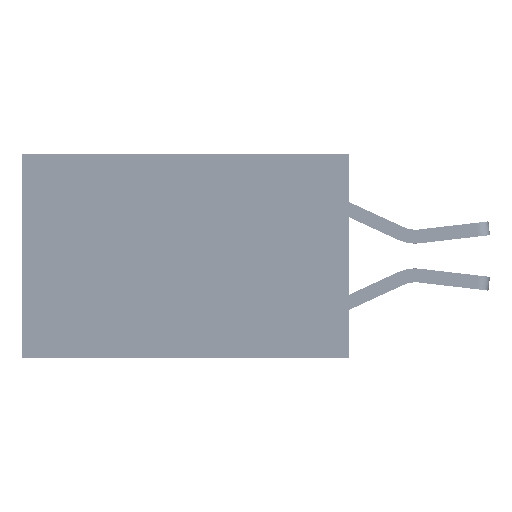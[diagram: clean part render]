
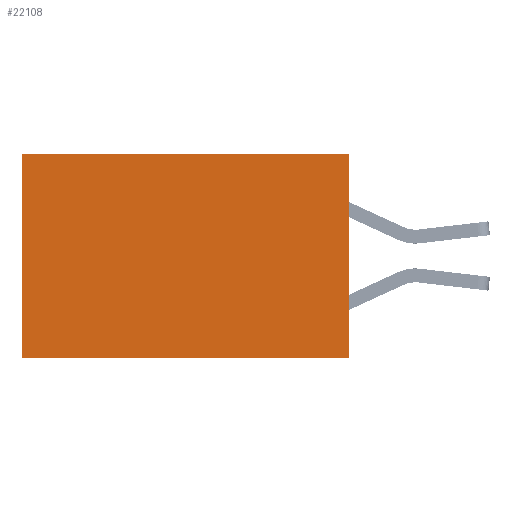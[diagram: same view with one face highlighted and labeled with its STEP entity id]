
A CAD part, left-side view. The second image highlights one B-rep face of the part: STEP entity #22108.
In plain terms, the highlighted planar face has unit normal (-1, 0, 0).
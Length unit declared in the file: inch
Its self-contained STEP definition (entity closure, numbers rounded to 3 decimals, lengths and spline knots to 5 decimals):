
#713 = CARTESIAN_POINT ( 'NONE',  ( 0.277, 0., -0.37 ) ) ;
#821 = DIRECTION ( 'NONE',  ( 0., 0., -1. ) ) ;
#1561 = CARTESIAN_POINT ( 'NONE',  ( 0.277, 0., 0. ) ) ;
#1711 = VERTEX_POINT ( 'NONE', #6669 ) ;
#3980 = CARTESIAN_POINT ( 'NONE',  ( 0.277, 0.59, 0. ) ) ;
#5219 = VECTOR ( 'NONE', #12526, 39.37008 ) ;
#6503 = PLANE ( 'NONE',  #19017 ) ;
#6669 = CARTESIAN_POINT ( 'NONE',  ( 0.277, 0., -0.37 ) ) ;
#7252 = EDGE_CURVE ( 'NONE', #13490, #1711, #30093, .T. ) ;
#7420 = CARTESIAN_POINT ( 'NONE',  ( 0.277, 0.59, -0.37 ) ) ;
#9092 = FACE_OUTER_BOUND ( 'NONE', #24923, .T. ) ;
#9891 = DIRECTION ( 'NONE',  ( 0., 1., 0. ) ) ;
#10445 = VECTOR ( 'NONE', #821, 39.37008 ) ;
#11364 = EDGE_CURVE ( 'NONE', #23473, #18302, #22721, .T. ) ;
#11895 = CARTESIAN_POINT ( 'NONE',  ( 0.277, 0., -0.37 ) ) ;
#12526 = DIRECTION ( 'NONE',  ( 0., 1., 0. ) ) ;
#13490 = VERTEX_POINT ( 'NONE', #15032 ) ;
#14504 = ORIENTED_EDGE ( 'NONE', *, *, #16308, .F. ) ;
#14604 = DIRECTION ( 'NONE',  ( 1., 0., 0. ) ) ;
#15032 = CARTESIAN_POINT ( 'NONE',  ( 0.277, 0., 0. ) ) ;
#16308 = EDGE_CURVE ( 'NONE', #1711, #18302, #29910, .T. ) ;
#16460 = ORIENTED_EDGE ( 'NONE', *, *, #7252, .F. ) ;
#16603 = VECTOR ( 'NONE', #9891, 39.37008 ) ;
#18302 = VERTEX_POINT ( 'NONE', #7420 ) ;
#19017 = AXIS2_PLACEMENT_3D ( 'NONE', #11895, #14604, #33185 ) ;
#20271 = CARTESIAN_POINT ( 'NONE',  ( 0.277, 0.59, -0.37 ) ) ;
#21160 = LINE ( 'NONE', #1561, #5219 ) ;
#22108 = ADVANCED_FACE ( 'NONE', ( #9092 ), #6503, .F. ) ;
#22721 = LINE ( 'NONE', #20271, #28971 ) ;
#23473 = VERTEX_POINT ( 'NONE', #3980 ) ;
#23625 = ORIENTED_EDGE ( 'NONE', *, *, #11364, .T. ) ;
#24923 = EDGE_LOOP ( 'NONE', ( #23625, #14504, #16460, #26257 ) ) ;
#25888 = CARTESIAN_POINT ( 'NONE',  ( 0.277, 0., -0.37 ) ) ;
#26257 = ORIENTED_EDGE ( 'NONE', *, *, #30333, .T. ) ;
#28971 = VECTOR ( 'NONE', #33500, 39.37008 ) ;
#29910 = LINE ( 'NONE', #25888, #16603 ) ;
#30093 = LINE ( 'NONE', #713, #10445 ) ;
#30333 = EDGE_CURVE ( 'NONE', #13490, #23473, #21160, .T. ) ;
#33185 = DIRECTION ( 'NONE',  ( 0., 0., -1. ) ) ;
#33500 = DIRECTION ( 'NONE',  ( 0., 0., -1. ) ) ;
